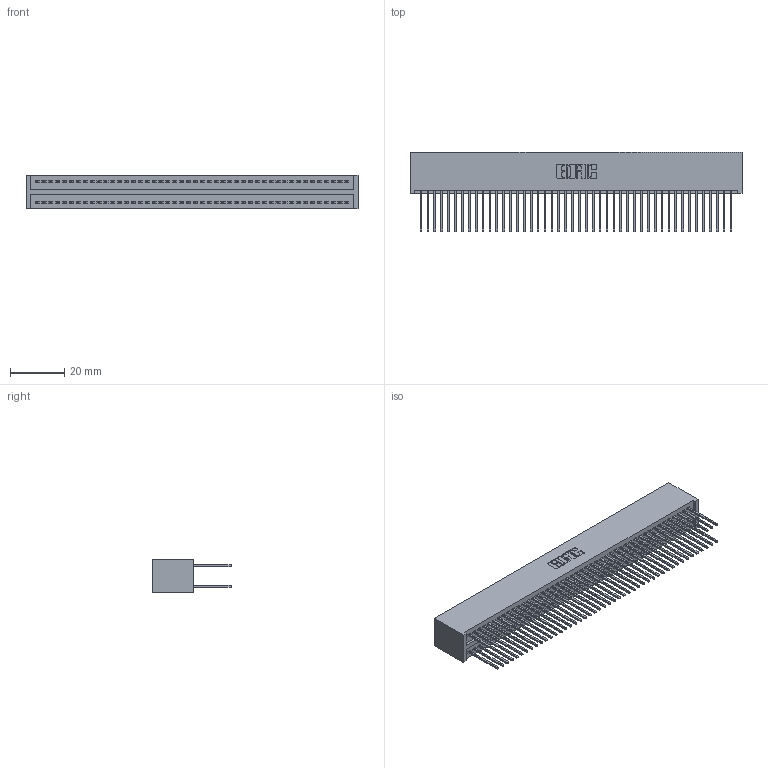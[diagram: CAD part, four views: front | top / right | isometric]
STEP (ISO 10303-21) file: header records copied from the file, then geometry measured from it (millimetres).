
FILE_DESCRIPTION (( 'STEP AP203' ), '1' );
FILE_NAME ('325-092-540-201.STEP', '2020-02-25T05:52:24', ( '' ), ( '' ), 'SwSTEP 2.0', 'SolidWorks 2016', '' );
FILE_SCHEMA (( 'CONFIG_CONTROL_DESIGN' ));
Length unit declared in the file: inch
Products named in the file (3): 325 Part_Lugless; 325-292-001_325-293-140; 325-092-540-201
Assembly tree (93 placements, depth 2):
  325-092-540-201
    325 Part_Lugless
    325-292-001_325-293-140  x92
Bounding box: 122.48 x 29.46 x 12.45 mm (x, y, z)
Volume: 16802.5 mm3; surface area: 22753.3 mm2
Topology: 93 solids, 93 shells, 4890 faces, 14547 edges, 9574 vertices
Faces by surface type: plane 3378, cylinder 1512
Entity records: 28817 total; most frequent: CARTESIAN_POINT 4770, ORIENTED_EDGE 4706, DIRECTION 4061, EDGE_CURVE 2353, VECTOR 2233, LINE 2233, VERTEX_POINT 1566, AXIS2_PLACEMENT_3D 914
